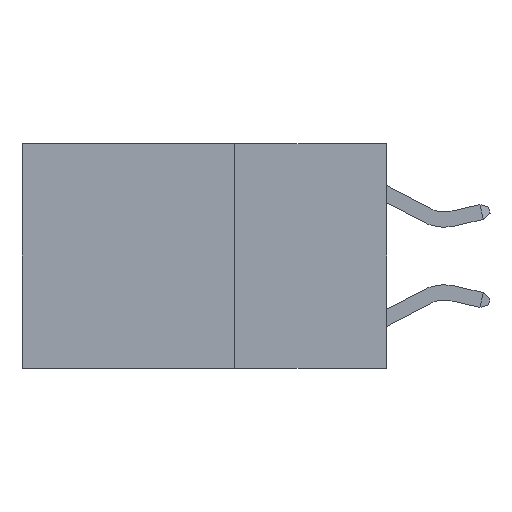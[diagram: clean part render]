
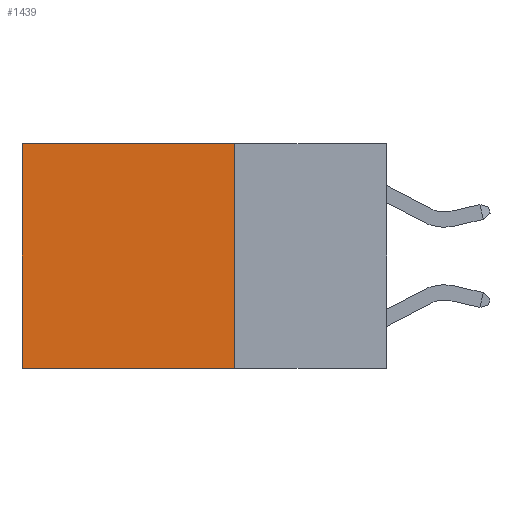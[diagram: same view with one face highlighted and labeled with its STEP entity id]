
A CAD part, left-side view. The second image highlights one B-rep face of the part: STEP entity #1439.
In plain terms, the highlighted planar face has unit normal (-1, 0, 0).
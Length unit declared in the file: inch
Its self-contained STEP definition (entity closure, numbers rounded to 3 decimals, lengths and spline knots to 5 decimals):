
#185 = DIRECTION ( 'NONE',  ( 0., 0., -1. ) ) ;
#477 = ORIENTED_EDGE ( 'NONE', *, *, #1271, .T. ) ;
#482 = DIRECTION ( 'NONE',  ( 0., 0., -1. ) ) ;
#1271 = EDGE_CURVE ( 'NONE', #6856, #9291, #2159, .T. ) ;
#1439 = ADVANCED_FACE ( 'NONE', ( #6572 ), #6285, .F. ) ;
#1742 = ORIENTED_EDGE ( 'NONE', *, *, #4016, .T. ) ;
#1854 = CARTESIAN_POINT ( 'NONE',  ( 0.2625, 0.6, -0.37 ) ) ;
#2159 = LINE ( 'NONE', #9005, #9654 ) ;
#2164 = EDGE_CURVE ( 'NONE', #2878, #9291, #2820, .T. ) ;
#2600 = DIRECTION ( 'NONE',  ( 0., 1., 0. ) ) ;
#2820 = LINE ( 'NONE', #5105, #5062 ) ;
#2878 = VERTEX_POINT ( 'NONE', #9173 ) ;
#3229 = CARTESIAN_POINT ( 'NONE',  ( 0.2625, 0.6, 0. ) ) ;
#3470 = EDGE_CURVE ( 'NONE', #5640, #2878, #5861, .T. ) ;
#3845 = VECTOR ( 'NONE', #185, 39.37008 ) ;
#4016 = EDGE_CURVE ( 'NONE', #5640, #6856, #5841, .T. ) ;
#5062 = VECTOR ( 'NONE', #7111, 39.37008 ) ;
#5105 = CARTESIAN_POINT ( 'NONE',  ( 0.2625, 0.25, -0.37 ) ) ;
#5640 = VERTEX_POINT ( 'NONE', #7409 ) ;
#5731 = CARTESIAN_POINT ( 'NONE',  ( 0.2625, 0.25, 0. ) ) ;
#5841 = LINE ( 'NONE', #5731, #7415 ) ;
#5861 = LINE ( 'NONE', #9401, #3845 ) ;
#6146 = DIRECTION ( 'NONE',  ( 0., 0., -1. ) ) ;
#6167 = DIRECTION ( 'NONE',  ( 1., 0., 0. ) ) ;
#6236 = ORIENTED_EDGE ( 'NONE', *, *, #2164, .F. ) ;
#6285 = PLANE ( 'NONE',  #8679 ) ;
#6420 = ORIENTED_EDGE ( 'NONE', *, *, #3470, .F. ) ;
#6572 = FACE_OUTER_BOUND ( 'NONE', #7446, .T. ) ;
#6824 = CARTESIAN_POINT ( 'NONE',  ( 0.2625, 0.25, 0. ) ) ;
#6856 = VERTEX_POINT ( 'NONE', #3229 ) ;
#7111 = DIRECTION ( 'NONE',  ( 0., 1., 0. ) ) ;
#7409 = CARTESIAN_POINT ( 'NONE',  ( 0.2625, 0.25, 0. ) ) ;
#7415 = VECTOR ( 'NONE', #2600, 39.37008 ) ;
#7446 = EDGE_LOOP ( 'NONE', ( #477, #6236, #6420, #1742 ) ) ;
#8679 = AXIS2_PLACEMENT_3D ( 'NONE', #6824, #6167, #6146 ) ;
#9005 = CARTESIAN_POINT ( 'NONE',  ( 0.2625, 0.6, 0. ) ) ;
#9173 = CARTESIAN_POINT ( 'NONE',  ( 0.2625, 0.25, -0.37 ) ) ;
#9291 = VERTEX_POINT ( 'NONE', #1854 ) ;
#9401 = CARTESIAN_POINT ( 'NONE',  ( 0.2625, 0.25, 0. ) ) ;
#9654 = VECTOR ( 'NONE', #482, 39.37008 ) ;
